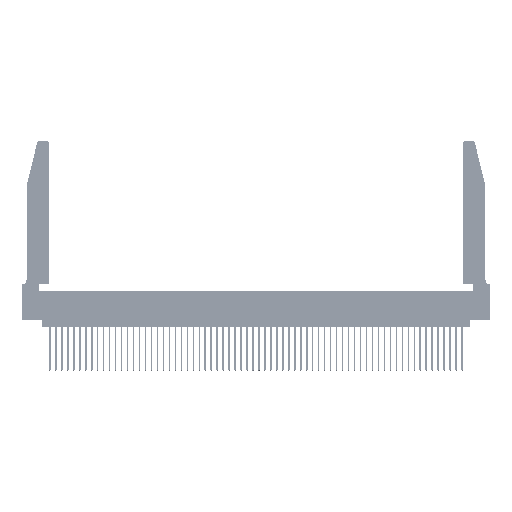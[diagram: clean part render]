
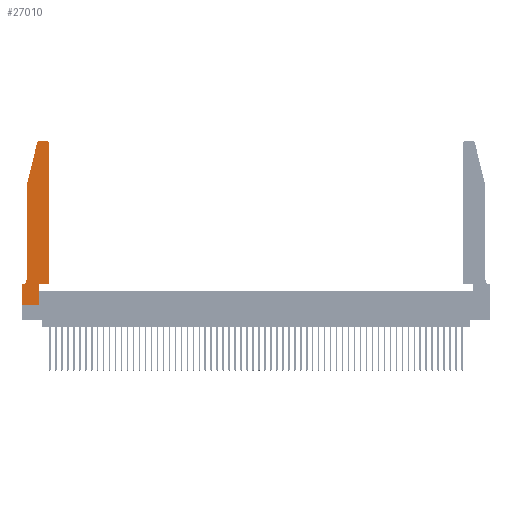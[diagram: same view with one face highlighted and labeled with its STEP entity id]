
A CAD part, top view. The second image highlights one B-rep face of the part: STEP entity #27010.
In plain terms, the highlighted planar face has unit normal (0, 0, 1).
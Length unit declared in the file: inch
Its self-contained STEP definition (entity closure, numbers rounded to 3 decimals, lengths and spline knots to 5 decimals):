
#95 = CARTESIAN_POINT ( 'NONE',  ( 0.4505, 0.35, 0.37 ) ) ;
#538 = CARTESIAN_POINT ( 'NONE',  ( 0.0755, 2., 0.37 ) ) ;
#711 = LINE ( 'NONE', #18361, #4061 ) ;
#3000 = LINE ( 'NONE', #27573, #32113 ) ;
#3275 = EDGE_CURVE ( 'NONE', #55291, #38899, #13404, .T. ) ;
#3642 = AXIS2_PLACEMENT_3D ( 'NONE', #28142, #40991, #32468 ) ;
#4061 = VECTOR ( 'NONE', #13630, 39.37008 ) ;
#4445 = CARTESIAN_POINT ( 'NONE',  ( 0.284, 2.75, 0.37 ) ) ;
#4580 = DIRECTION ( 'NONE',  ( -1., 0., 0. ) ) ;
#5051 = DIRECTION ( 'NONE',  ( 0., 0., 1. ) ) ;
#5900 = CARTESIAN_POINT ( 'NONE',  ( 0.0755, 0.42, 0.37 ) ) ;
#6137 = LINE ( 'NONE', #538, #54219 ) ;
#6520 = CARTESIAN_POINT ( 'NONE',  ( 0., 0., 0.37 ) ) ;
#6739 = AXIS2_PLACEMENT_3D ( 'NONE', #51737, #33899, #47174 ) ;
#6790 = ORIENTED_EDGE ( 'NONE', *, *, #19413, .T. ) ;
#7356 = VERTEX_POINT ( 'NONE', #14427 ) ;
#7949 = EDGE_CURVE ( 'NONE', #16000, #7356, #711, .T. ) ;
#8589 = CARTESIAN_POINT ( 'NONE',  ( 0.0755, 2., 0.37 ) ) ;
#9953 = VECTOR ( 'NONE', #49744, 39.37008 ) ;
#9966 = VERTEX_POINT ( 'NONE', #5900 ) ;
#10173 = CARTESIAN_POINT ( 'NONE',  ( 0.0755, 2., 0.37 ) ) ;
#11111 = ORIENTED_EDGE ( 'NONE', *, *, #54410, .T. ) ;
#13085 = AXIS2_PLACEMENT_3D ( 'NONE', #27896, #49675, #32588 ) ;
#13313 = DIRECTION ( 'NONE',  ( 1., 0., 0. ) ) ;
#13404 = LINE ( 'NONE', #55070, #41108 ) ;
#13630 = DIRECTION ( 'NONE',  ( 0., 1., 0. ) ) ;
#14079 = VECTOR ( 'NONE', #13313, 39.37008 ) ;
#14129 = LINE ( 'NONE', #95, #14079 ) ;
#14273 = DIRECTION ( 'NONE',  ( 1., 0., 0. ) ) ;
#14427 = CARTESIAN_POINT ( 'NONE',  ( 0.2865, 0.35, 0.37 ) ) ;
#14545 = LINE ( 'NONE', #44288, #47148 ) ;
#16000 = VERTEX_POINT ( 'NONE', #25293 ) ;
#16560 = CARTESIAN_POINT ( 'NONE',  ( 0.4505, 0.35, 0.37 ) ) ;
#16631 = VERTEX_POINT ( 'NONE', #47547 ) ;
#16769 = LINE ( 'NONE', #30511, #30360 ) ;
#16989 = CARTESIAN_POINT ( 'NONE',  ( 0.0055, 0.35, 0.37 ) ) ;
#17425 = EDGE_CURVE ( 'NONE', #21766, #39258, #6137, .T. ) ;
#17664 = DIRECTION ( 'NONE',  ( 0., 1., 0. ) ) ;
#18361 = CARTESIAN_POINT ( 'NONE',  ( 0.2865, 0.35, 0.37 ) ) ;
#18519 = EDGE_CURVE ( 'NONE', #16631, #36416, #16769, .T. ) ;
#18607 = VECTOR ( 'NONE', #17664, 39.37008 ) ;
#19413 = EDGE_CURVE ( 'NONE', #39258, #9966, #51968, .T. ) ;
#20893 = ORIENTED_EDGE ( 'NONE', *, *, #34680, .T. ) ;
#21692 = EDGE_CURVE ( 'NONE', #9966, #44967, #37098, .T. ) ;
#21765 = ORIENTED_EDGE ( 'NONE', *, *, #18519, .T. ) ;
#21766 = VERTEX_POINT ( 'NONE', #41550 ) ;
#22087 = ORIENTED_EDGE ( 'NONE', *, *, #21692, .T. ) ;
#25293 = CARTESIAN_POINT ( 'NONE',  ( 0.2865, 0., 0.37 ) ) ;
#25398 = LINE ( 'NONE', #30386, #18607 ) ;
#25466 = VERTEX_POINT ( 'NONE', #30965 ) ;
#26086 = CIRCLE ( 'NONE', #56083, 0.03 ) ;
#27010 = ADVANCED_FACE ( 'NONE', ( #40601 ), #29555, .T. ) ;
#27573 = CARTESIAN_POINT ( 'NONE',  ( 0., 0., 0.37 ) ) ;
#27896 = CARTESIAN_POINT ( 'NONE',  ( 0.284, 2.72, 0.37 ) ) ;
#28142 = CARTESIAN_POINT ( 'NONE',  ( 0.0055, 0.42, 0.37 ) ) ;
#28334 = ORIENTED_EDGE ( 'NONE', *, *, #50266, .T. ) ;
#28814 = ORIENTED_EDGE ( 'NONE', *, *, #3275, .T. ) ;
#29555 = PLANE ( 'NONE',  #6739 ) ;
#30263 = ORIENTED_EDGE ( 'NONE', *, *, #30861, .T. ) ;
#30360 = VECTOR ( 'NONE', #4580, 39.37008 ) ;
#30386 = CARTESIAN_POINT ( 'NONE',  ( 0.4505, 0.35, 0.37 ) ) ;
#30511 = CARTESIAN_POINT ( 'NONE',  ( 0.2605, 2.75, 0.37 ) ) ;
#30861 = EDGE_CURVE ( 'NONE', #38899, #16000, #3000, .T. ) ;
#30965 = CARTESIAN_POINT ( 'NONE',  ( 0.4505, 2.72, 0.37 ) ) ;
#30975 = CARTESIAN_POINT ( 'NONE',  ( 0.4205, 2.72, 0.37 ) ) ;
#31357 = DIRECTION ( 'NONE',  ( 1., 0., 0. ) ) ;
#32113 = VECTOR ( 'NONE', #31357, 39.37008 ) ;
#32468 = DIRECTION ( 'NONE',  ( -1., 0., 0. ) ) ;
#32588 = DIRECTION ( 'NONE',  ( 1., 0., 0. ) ) ;
#33899 = DIRECTION ( 'NONE',  ( 0., 0., 1. ) ) ;
#34680 = EDGE_CURVE ( 'NONE', #7356, #48907, #14129, .T. ) ;
#34866 = EDGE_CURVE ( 'NONE', #36416, #21766, #39387, .T. ) ;
#36416 = VERTEX_POINT ( 'NONE', #4445 ) ;
#36802 = CARTESIAN_POINT ( 'NONE',  ( 0., 0.35, 0.37 ) ) ;
#37098 = CIRCLE ( 'NONE', #3642, 0.07 ) ;
#38279 = ORIENTED_EDGE ( 'NONE', *, *, #38864, .T. ) ;
#38459 = EDGE_LOOP ( 'NONE', ( #21765, #48047, #54896, #6790, #22087, #11111, #28814, #30263, #38956, #20893, #28334, #38279 ) ) ;
#38864 = EDGE_CURVE ( 'NONE', #25466, #16631, #26086, .T. ) ;
#38899 = VERTEX_POINT ( 'NONE', #6520 ) ;
#38956 = ORIENTED_EDGE ( 'NONE', *, *, #7949, .T. ) ;
#39258 = VERTEX_POINT ( 'NONE', #8589 ) ;
#39387 = CIRCLE ( 'NONE', #13085, 0.03 ) ;
#40601 = FACE_OUTER_BOUND ( 'NONE', #38459, .T. ) ;
#40991 = DIRECTION ( 'NONE',  ( 0., 0., -1. ) ) ;
#41108 = VECTOR ( 'NONE', #42129, 39.37008 ) ;
#41550 = CARTESIAN_POINT ( 'NONE',  ( 0.25487, 2.72718, 0.37 ) ) ;
#42129 = DIRECTION ( 'NONE',  ( 0., -1., 0. ) ) ;
#44288 = CARTESIAN_POINT ( 'NONE',  ( 0.0755, 0.35, 0.37 ) ) ;
#44967 = VERTEX_POINT ( 'NONE', #16989 ) ;
#47148 = VECTOR ( 'NONE', #49227, 39.37008 ) ;
#47174 = DIRECTION ( 'NONE',  ( 1., 0., 0. ) ) ;
#47547 = CARTESIAN_POINT ( 'NONE',  ( 0.4205, 2.75, 0.37 ) ) ;
#48047 = ORIENTED_EDGE ( 'NONE', *, *, #34866, .T. ) ;
#48907 = VERTEX_POINT ( 'NONE', #16560 ) ;
#49227 = DIRECTION ( 'NONE',  ( -1., 0., 0. ) ) ;
#49675 = DIRECTION ( 'NONE',  ( 0., 0., 1. ) ) ;
#49744 = DIRECTION ( 'NONE',  ( 0., -1., 0. ) ) ;
#50266 = EDGE_CURVE ( 'NONE', #48907, #25466, #25398, .T. ) ;
#51737 = CARTESIAN_POINT ( 'NONE',  ( 0., 0.35, 0.37 ) ) ;
#51968 = LINE ( 'NONE', #10173, #9953 ) ;
#52058 = DIRECTION ( 'NONE',  ( -0.239, -0.971, 0. ) ) ;
#54219 = VECTOR ( 'NONE', #52058, 39.37008 ) ;
#54410 = EDGE_CURVE ( 'NONE', #44967, #55291, #14545, .T. ) ;
#54896 = ORIENTED_EDGE ( 'NONE', *, *, #17425, .T. ) ;
#55070 = CARTESIAN_POINT ( 'NONE',  ( 0., 0., 0.37 ) ) ;
#55291 = VERTEX_POINT ( 'NONE', #36802 ) ;
#56083 = AXIS2_PLACEMENT_3D ( 'NONE', #30975, #5051, #14273 ) ;
